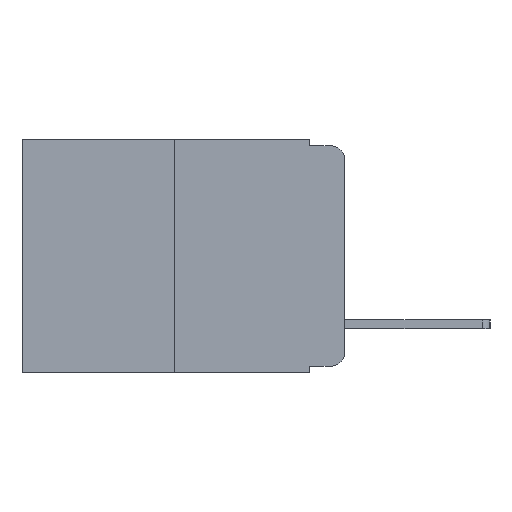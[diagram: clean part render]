
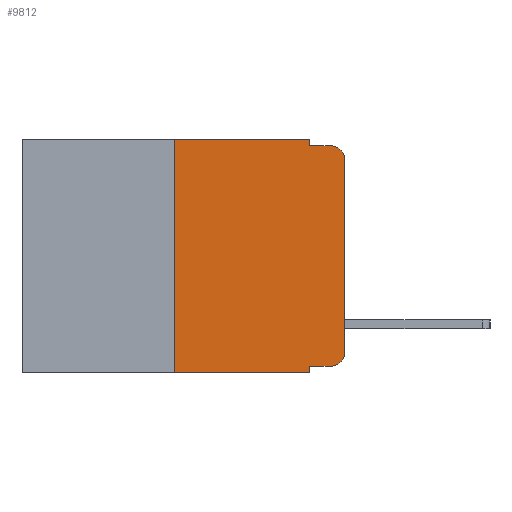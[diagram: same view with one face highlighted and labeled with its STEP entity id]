
A CAD part, left-side view. The second image highlights one B-rep face of the part: STEP entity #9812.
In plain terms, the highlighted planar face has unit normal (-1, 0, 0).
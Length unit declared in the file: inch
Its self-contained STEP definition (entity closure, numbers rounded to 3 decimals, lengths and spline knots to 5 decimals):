
#80 = VERTEX_POINT ( 'NONE', #2430 ) ;
#894 = CARTESIAN_POINT ( 'NONE',  ( 0., 0., -0.03 ) ) ;
#1082 = ORIENTED_EDGE ( 'NONE', *, *, #18457, .F. ) ;
#1106 = AXIS2_PLACEMENT_3D ( 'NONE', #8855, #19087, #10340 ) ;
#1109 = DIRECTION ( 'NONE',  ( 0., 0., -1. ) ) ;
#1257 = EDGE_CURVE ( 'NONE', #2665, #12734, #13690, .T. ) ;
#1260 = DIRECTION ( 'NONE',  ( 0., -1., 0. ) ) ;
#1973 = VERTEX_POINT ( 'NONE', #11697 ) ;
#2320 = AXIS2_PLACEMENT_3D ( 'NONE', #6581, #16945, #8068 ) ;
#2419 = LINE ( 'NONE', #2848, #10127 ) ;
#2430 = CARTESIAN_POINT ( 'NONE',  ( 0., 0., -0.313 ) ) ;
#2647 = VERTEX_POINT ( 'NONE', #7042 ) ;
#2665 = VERTEX_POINT ( 'NONE', #17393 ) ;
#2848 = CARTESIAN_POINT ( 'NONE',  ( 0., 0.051, 0. ) ) ;
#3589 = CARTESIAN_POINT ( 'NONE',  ( 0., 0.051, -0.333 ) ) ;
#3604 = ORIENTED_EDGE ( 'NONE', *, *, #17869, .T. ) ;
#4213 = CARTESIAN_POINT ( 'NONE',  ( 0., 0.051, 0. ) ) ;
#4333 = LINE ( 'NONE', #18047, #7434 ) ;
#4691 = LINE ( 'NONE', #16202, #8264 ) ;
#4836 = LINE ( 'NONE', #15032, #12835 ) ;
#5145 = ORIENTED_EDGE ( 'NONE', *, *, #1257, .F. ) ;
#5185 = EDGE_CURVE ( 'NONE', #9771, #7193, #16445, .T. ) ;
#5399 = CARTESIAN_POINT ( 'NONE',  ( 0., 0.051, -0.343 ) ) ;
#6209 = EDGE_CURVE ( 'NONE', #80, #9771, #11770, .T. ) ;
#6279 = LINE ( 'NONE', #17723, #9303 ) ;
#6581 = CARTESIAN_POINT ( 'NONE',  ( 0., 0.02, -0.313 ) ) ;
#6604 = EDGE_CURVE ( 'NONE', #11271, #1973, #4691, .T. ) ;
#6782 = CARTESIAN_POINT ( 'NONE',  ( 0., 0.25, -0.343 ) ) ;
#7042 = CARTESIAN_POINT ( 'NONE',  ( 0., 0.051, -0.01 ) ) ;
#7193 = VERTEX_POINT ( 'NONE', #15993 ) ;
#7194 = VECTOR ( 'NONE', #11233, 39.37008 ) ;
#7322 = PLANE ( 'NONE',  #1106 ) ;
#7347 = DIRECTION ( 'NONE',  ( 0., -1., 0. ) ) ;
#7434 = VECTOR ( 'NONE', #9215, 39.37008 ) ;
#8068 = DIRECTION ( 'NONE',  ( 0., 0., -1. ) ) ;
#8264 = VECTOR ( 'NONE', #17655, 39.37008 ) ;
#8607 = EDGE_CURVE ( 'NONE', #14608, #2647, #2419, .T. ) ;
#8855 = CARTESIAN_POINT ( 'NONE',  ( 0., 0.473, 0. ) ) ;
#9215 = DIRECTION ( 'NONE',  ( 0., -1., 0. ) ) ;
#9303 = VECTOR ( 'NONE', #7347, 39.37008 ) ;
#9616 = CARTESIAN_POINT ( 'NONE',  ( 0., 0.02, -0.333 ) ) ;
#9771 = VERTEX_POINT ( 'NONE', #894 ) ;
#9812 = ADVANCED_FACE ( 'NONE', ( #11472 ), #7322, .F. ) ;
#10127 = VECTOR ( 'NONE', #15007, 39.37008 ) ;
#10340 = DIRECTION ( 'NONE',  ( 0., 0., -1. ) ) ;
#10393 = DIRECTION ( 'NONE',  ( -1., 0., 0. ) ) ;
#10435 = EDGE_LOOP ( 'NONE', ( #14522, #18343, #1082, #13837, #17691, #19447, #12662, #5145, #18106, #3604 ) ) ;
#11233 = DIRECTION ( 'NONE',  ( 0., -1., 0. ) ) ;
#11271 = VERTEX_POINT ( 'NONE', #6782 ) ;
#11472 = FACE_OUTER_BOUND ( 'NONE', #10435, .T. ) ;
#11697 = CARTESIAN_POINT ( 'NONE',  ( 0., 0.25, 0. ) ) ;
#11770 = LINE ( 'NONE', #18987, #19057 ) ;
#12127 = VERTEX_POINT ( 'NONE', #9616 ) ;
#12662 = ORIENTED_EDGE ( 'NONE', *, *, #14645, .T. ) ;
#12734 = VERTEX_POINT ( 'NONE', #5399 ) ;
#12835 = VECTOR ( 'NONE', #1260, 39.37008 ) ;
#13214 = VECTOR ( 'NONE', #15119, 39.37008 ) ;
#13250 = DIRECTION ( 'NONE',  ( 0., 0., 1. ) ) ;
#13690 = LINE ( 'NONE', #15033, #13214 ) ;
#13837 = ORIENTED_EDGE ( 'NONE', *, *, #8607, .F. ) ;
#14522 = ORIENTED_EDGE ( 'NONE', *, *, #6209, .T. ) ;
#14608 = VERTEX_POINT ( 'NONE', #4213 ) ;
#14645 = EDGE_CURVE ( 'NONE', #11271, #12734, #6279, .T. ) ;
#15007 = DIRECTION ( 'NONE',  ( 0., 0., -1. ) ) ;
#15032 = CARTESIAN_POINT ( 'NONE',  ( 0., 0.051, -0.01 ) ) ;
#15033 = CARTESIAN_POINT ( 'NONE',  ( 0., 0.051, 0. ) ) ;
#15119 = DIRECTION ( 'NONE',  ( 0., 0., -1. ) ) ;
#15993 = CARTESIAN_POINT ( 'NONE',  ( 0., 0.02, -0.01 ) ) ;
#16202 = CARTESIAN_POINT ( 'NONE',  ( 0., 0.25, 0. ) ) ;
#16445 = CIRCLE ( 'NONE', #18626, 0.02 ) ;
#16945 = DIRECTION ( 'NONE',  ( -1., 0., 0. ) ) ;
#17393 = CARTESIAN_POINT ( 'NONE',  ( 0., 0.051, -0.333 ) ) ;
#17655 = DIRECTION ( 'NONE',  ( 0., 0., 1. ) ) ;
#17662 = CIRCLE ( 'NONE', #2320, 0.02 ) ;
#17691 = ORIENTED_EDGE ( 'NONE', *, *, #18533, .F. ) ;
#17723 = CARTESIAN_POINT ( 'NONE',  ( 0., 0.473, -0.343 ) ) ;
#17869 = EDGE_CURVE ( 'NONE', #12127, #80, #17662, .T. ) ;
#18047 = CARTESIAN_POINT ( 'NONE',  ( 0., 0.473, 0. ) ) ;
#18060 = LINE ( 'NONE', #3589, #7194 ) ;
#18106 = ORIENTED_EDGE ( 'NONE', *, *, #18800, .T. ) ;
#18343 = ORIENTED_EDGE ( 'NONE', *, *, #5185, .T. ) ;
#18457 = EDGE_CURVE ( 'NONE', #2647, #7193, #4836, .T. ) ;
#18533 = EDGE_CURVE ( 'NONE', #1973, #14608, #4333, .T. ) ;
#18626 = AXIS2_PLACEMENT_3D ( 'NONE', #19145, #10393, #1109 ) ;
#18800 = EDGE_CURVE ( 'NONE', #2665, #12127, #18060, .T. ) ;
#18987 = CARTESIAN_POINT ( 'NONE',  ( 0., 0., 0. ) ) ;
#19057 = VECTOR ( 'NONE', #13250, 39.37008 ) ;
#19087 = DIRECTION ( 'NONE',  ( 1., 0., 0. ) ) ;
#19145 = CARTESIAN_POINT ( 'NONE',  ( 0., 0.02, -0.03 ) ) ;
#19447 = ORIENTED_EDGE ( 'NONE', *, *, #6604, .F. ) ;
